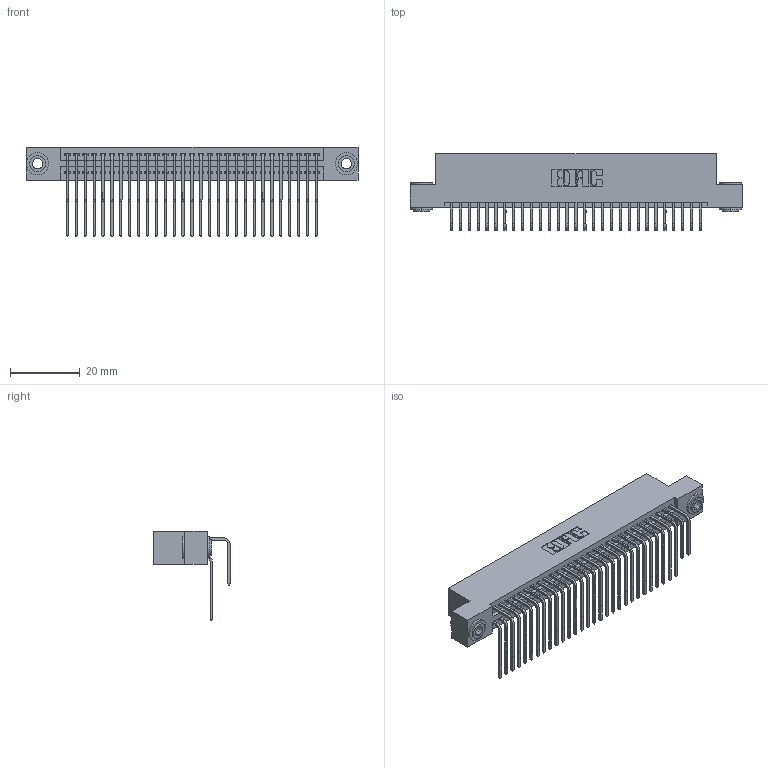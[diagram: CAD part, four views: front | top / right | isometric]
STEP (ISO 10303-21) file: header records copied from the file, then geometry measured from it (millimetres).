
FILE_DESCRIPTION (( 'STEP AP203' ), '1' );
FILE_NAME ('345-058-558-203.STEP', '2019-10-30T06:14:11', ( '' ), ( '' ), 'SwSTEP 2.0', 'SolidWorks 2016', '' );
FILE_SCHEMA (( 'CONFIG_CONTROL_DESIGN' ));
Length unit declared in the file: inch
Products named in the file (5): 345-058-558-203; 345 Part_Flush Mounting Lugs - 0.156 Dia-TH; 345-250-002_345-250-002-102; 345-292-001_558 559 Tail - 1; 345-292-001_558 Tail - 2
Assembly tree (61 placements, depth 2):
  345-058-558-203
    345 Part_Flush Mounting Lugs - 0.156 Dia-TH
    345-292-001_558 559 Tail - 1  x29
    345-292-001_558 Tail - 2  x29
    345-250-002_345-250-002-102  x2
Bounding box: 94.87 x 21.83 x 25.53 mm (x, y, z)
Volume: 9449 mm3; surface area: 15493.6 mm2
Topology: 61 solids, 61 shells, 3180 faces, 9407 edges, 6190 vertices
Faces by surface type: plane 2120, cylinder 1052, cone 8
Entity records: 26806 total; most frequent: CARTESIAN_POINT 4526, ORIENTED_EDGE 4402, DIRECTION 4011, EDGE_CURVE 2201, VECTOR 1889, LINE 1889, VERTEX_POINT 1462, AXIS2_PLACEMENT_3D 1061
